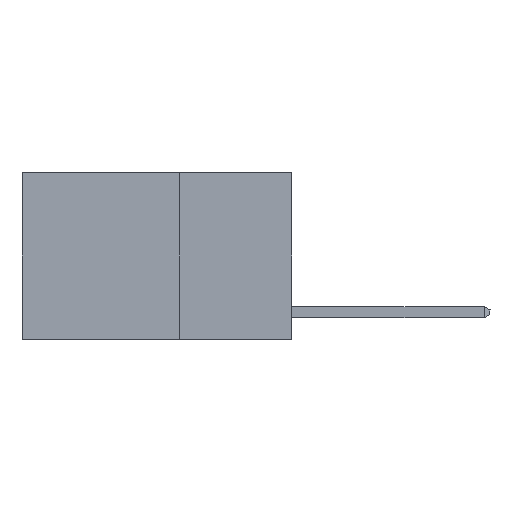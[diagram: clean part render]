
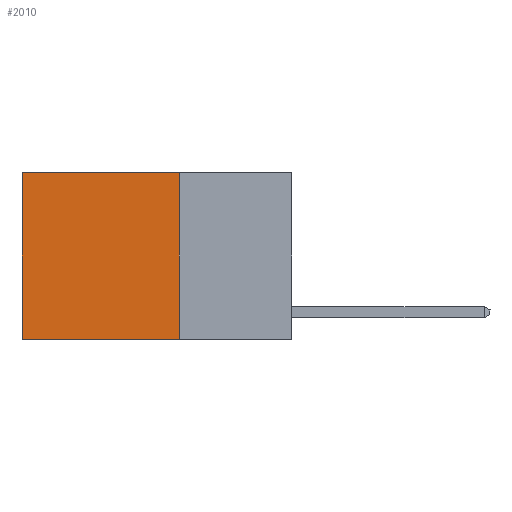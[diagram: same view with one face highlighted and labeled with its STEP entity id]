
A CAD part, left-side view. The second image highlights one B-rep face of the part: STEP entity #2010.
In plain terms, the highlighted planar face has unit normal (-1, 0, 0).
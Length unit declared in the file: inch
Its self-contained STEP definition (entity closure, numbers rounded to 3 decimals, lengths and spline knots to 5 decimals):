
#131 = VECTOR ( 'NONE', #8715, 39.37008 ) ;
#1263 = VERTEX_POINT ( 'NONE', #12203 ) ;
#1387 = CARTESIAN_POINT ( 'NONE',  ( 0.2625, 0.25, 0. ) ) ;
#1996 = DIRECTION ( 'NONE',  ( 0., 1., 0. ) ) ;
#2010 = ADVANCED_FACE ( 'NONE', ( #8634 ), #10120, .F. ) ;
#2644 = CARTESIAN_POINT ( 'NONE',  ( 0.2625, 0.6, 0. ) ) ;
#2862 = CARTESIAN_POINT ( 'NONE',  ( 0.2625, 0.25, 0. ) ) ;
#3137 = ORIENTED_EDGE ( 'NONE', *, *, #7756, .F. ) ;
#3149 = DIRECTION ( 'NONE',  ( 0., 1., 0. ) ) ;
#3439 = DIRECTION ( 'NONE',  ( 0., 0., -1. ) ) ;
#3888 = CARTESIAN_POINT ( 'NONE',  ( 0.2625, 0.6, -0.37 ) ) ;
#4067 = EDGE_CURVE ( 'NONE', #12293, #1263, #9171, .T. ) ;
#4356 = ORIENTED_EDGE ( 'NONE', *, *, #9046, .F. ) ;
#4444 = AXIS2_PLACEMENT_3D ( 'NONE', #1387, #9219, #3439 ) ;
#4777 = VERTEX_POINT ( 'NONE', #3888 ) ;
#5531 = LINE ( 'NONE', #11350, #9620 ) ;
#6132 = CARTESIAN_POINT ( 'NONE',  ( 0.2625, 0.25, -0.37 ) ) ;
#6183 = EDGE_LOOP ( 'NONE', ( #8527, #3137, #4356, #7019 ) ) ;
#6957 = EDGE_CURVE ( 'NONE', #1263, #4777, #7607, .T. ) ;
#7019 = ORIENTED_EDGE ( 'NONE', *, *, #4067, .T. ) ;
#7607 = LINE ( 'NONE', #2644, #8214 ) ;
#7756 = EDGE_CURVE ( 'NONE', #7990, #4777, #5531, .T. ) ;
#7819 = CARTESIAN_POINT ( 'NONE',  ( 0.2625, 0.25, 0. ) ) ;
#7990 = VERTEX_POINT ( 'NONE', #6132 ) ;
#8214 = VECTOR ( 'NONE', #12436, 39.37008 ) ;
#8527 = ORIENTED_EDGE ( 'NONE', *, *, #6957, .T. ) ;
#8634 = FACE_OUTER_BOUND ( 'NONE', #6183, .T. ) ;
#8715 = DIRECTION ( 'NONE',  ( 0., 0., -1. ) ) ;
#8875 = VECTOR ( 'NONE', #1996, 39.37008 ) ;
#9046 = EDGE_CURVE ( 'NONE', #12293, #7990, #11460, .T. ) ;
#9171 = LINE ( 'NONE', #7819, #8875 ) ;
#9219 = DIRECTION ( 'NONE',  ( 1., 0., 0. ) ) ;
#9620 = VECTOR ( 'NONE', #3149, 39.37008 ) ;
#10120 = PLANE ( 'NONE',  #4444 ) ;
#11350 = CARTESIAN_POINT ( 'NONE',  ( 0.2625, 0.25, -0.37 ) ) ;
#11460 = LINE ( 'NONE', #2862, #131 ) ;
#12203 = CARTESIAN_POINT ( 'NONE',  ( 0.2625, 0.6, 0. ) ) ;
#12293 = VERTEX_POINT ( 'NONE', #12410 ) ;
#12410 = CARTESIAN_POINT ( 'NONE',  ( 0.2625, 0.25, 0. ) ) ;
#12436 = DIRECTION ( 'NONE',  ( 0., 0., -1. ) ) ;
